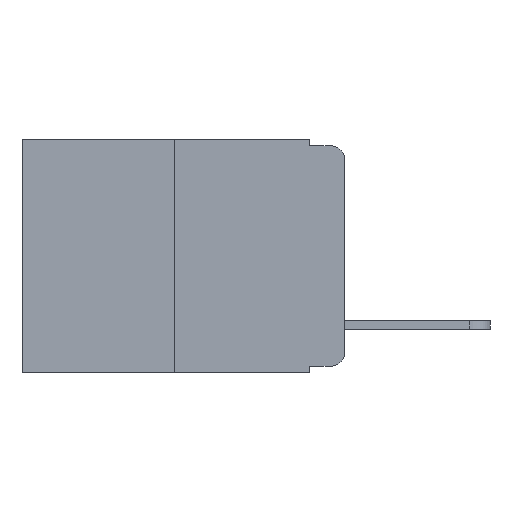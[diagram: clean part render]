
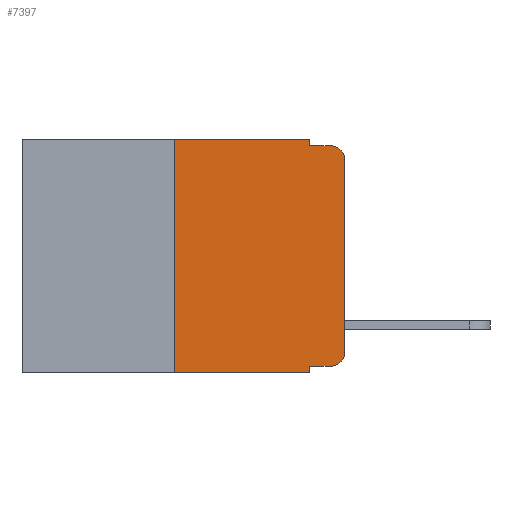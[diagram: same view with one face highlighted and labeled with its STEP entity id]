
A CAD part, left-side view. The second image highlights one B-rep face of the part: STEP entity #7397.
In plain terms, the highlighted planar face has unit normal (-1, 0, 0).
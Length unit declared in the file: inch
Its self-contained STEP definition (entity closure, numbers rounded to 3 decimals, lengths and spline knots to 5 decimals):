
#75 = LINE ( 'NONE', #168, #11359 ) ;
#168 = CARTESIAN_POINT ( 'NONE',  ( 0., 0.051, -0.333 ) ) ;
#244 = LINE ( 'NONE', #7957, #292 ) ;
#292 = VECTOR ( 'NONE', #8875, 39.37008 ) ;
#838 = VERTEX_POINT ( 'NONE', #10500 ) ;
#1460 = CARTESIAN_POINT ( 'NONE',  ( 0., 0., -0.313 ) ) ;
#1506 = EDGE_CURVE ( 'NONE', #4742, #7290, #4021, .T. ) ;
#1530 = ORIENTED_EDGE ( 'NONE', *, *, #1506, .T. ) ;
#1677 = ORIENTED_EDGE ( 'NONE', *, *, #1721, .T. ) ;
#1721 = EDGE_CURVE ( 'NONE', #7290, #1824, #3068, .T. ) ;
#1792 = ORIENTED_EDGE ( 'NONE', *, *, #2187, .F. ) ;
#1824 = VERTEX_POINT ( 'NONE', #8530 ) ;
#1874 = ORIENTED_EDGE ( 'NONE', *, *, #3678, .F. ) ;
#1945 = VERTEX_POINT ( 'NONE', #7128 ) ;
#1967 = ORIENTED_EDGE ( 'NONE', *, *, #5667, .F. ) ;
#2128 = ORIENTED_EDGE ( 'NONE', *, *, #4092, .F. ) ;
#2187 = EDGE_CURVE ( 'NONE', #7816, #1824, #11665, .T. ) ;
#2367 = ORIENTED_EDGE ( 'NONE', *, *, #3407, .T. ) ;
#2458 = ORIENTED_EDGE ( 'NONE', *, *, #4183, .F. ) ;
#2463 = CARTESIAN_POINT ( 'NONE',  ( 0., 0.051, 0. ) ) ;
#2758 = ORIENTED_EDGE ( 'NONE', *, *, #4461, .T. ) ;
#2759 = DIRECTION ( 'NONE',  ( -1., 0., 0. ) ) ;
#2853 = ORIENTED_EDGE ( 'NONE', *, *, #4691, .T. ) ;
#2864 = VECTOR ( 'NONE', #7560, 39.37008 ) ;
#3068 = CIRCLE ( 'NONE', #10586, 0.02 ) ;
#3407 = EDGE_CURVE ( 'NONE', #5128, #838, #244, .T. ) ;
#3635 = VECTOR ( 'NONE', #12746, 39.37008 ) ;
#3678 = EDGE_CURVE ( 'NONE', #10575, #7816, #6460, .T. ) ;
#3690 = VERTEX_POINT ( 'NONE', #12402 ) ;
#3712 = DIRECTION ( 'NONE',  ( 0., 0., 1. ) ) ;
#3852 = CARTESIAN_POINT ( 'NONE',  ( 0., 0.051, -0.01 ) ) ;
#4005 = VECTOR ( 'NONE', #10206, 39.37008 ) ;
#4021 = LINE ( 'NONE', #9619, #4005 ) ;
#4092 = EDGE_CURVE ( 'NONE', #5128, #6101, #4335, .T. ) ;
#4183 = EDGE_CURVE ( 'NONE', #1945, #838, #8688, .T. ) ;
#4283 = VECTOR ( 'NONE', #9826, 39.37008 ) ;
#4335 = LINE ( 'NONE', #7311, #4657 ) ;
#4381 = DIRECTION ( 'NONE',  ( 0., 0., -1. ) ) ;
#4461 = EDGE_CURVE ( 'NONE', #1945, #3690, #75, .T. ) ;
#4657 = VECTOR ( 'NONE', #3712, 39.37008 ) ;
#4691 = EDGE_CURVE ( 'NONE', #3690, #4742, #9610, .T. ) ;
#4742 = VERTEX_POINT ( 'NONE', #1460 ) ;
#4970 = CARTESIAN_POINT ( 'NONE',  ( 0., 0.25, -0.343 ) ) ;
#5128 = VERTEX_POINT ( 'NONE', #4970 ) ;
#5667 = EDGE_CURVE ( 'NONE', #6101, #10575, #9877, .T. ) ;
#6101 = VERTEX_POINT ( 'NONE', #12048 ) ;
#6220 = EDGE_LOOP ( 'NONE', ( #1530, #1677, #1792, #1874, #1967, #2128, #2367, #2458, #2758, #2853 ) ) ;
#6311 = AXIS2_PLACEMENT_3D ( 'NONE', #10920, #2759, #4381 ) ;
#6451 = DIRECTION ( 'NONE',  ( 0., -1., 0. ) ) ;
#6460 = LINE ( 'NONE', #2463, #3635 ) ;
#7128 = CARTESIAN_POINT ( 'NONE',  ( 0., 0.051, -0.333 ) ) ;
#7256 = DIRECTION ( 'NONE',  ( 0., -1., 0. ) ) ;
#7290 = VERTEX_POINT ( 'NONE', #12981 ) ;
#7311 = CARTESIAN_POINT ( 'NONE',  ( 0., 0.25, 0. ) ) ;
#7397 = ADVANCED_FACE ( 'NONE', ( #7904 ), #11223, .F. ) ;
#7560 = DIRECTION ( 'NONE',  ( 0., 0., -1. ) ) ;
#7816 = VERTEX_POINT ( 'NONE', #3852 ) ;
#7904 = FACE_OUTER_BOUND ( 'NONE', #6220, .T. ) ;
#7957 = CARTESIAN_POINT ( 'NONE',  ( 0., 0.473, -0.343 ) ) ;
#8482 = DIRECTION ( 'NONE',  ( 0., 0., -1. ) ) ;
#8486 = DIRECTION ( 'NONE',  ( -1., 0., 0. ) ) ;
#8530 = CARTESIAN_POINT ( 'NONE',  ( 0., 0.02, -0.01 ) ) ;
#8688 = LINE ( 'NONE', #9442, #2864 ) ;
#8875 = DIRECTION ( 'NONE',  ( 0., -1., 0. ) ) ;
#9058 = CARTESIAN_POINT ( 'NONE',  ( 0., 0.02, -0.03 ) ) ;
#9442 = CARTESIAN_POINT ( 'NONE',  ( 0., 0.051, 0. ) ) ;
#9610 = CIRCLE ( 'NONE', #6311, 0.02 ) ;
#9619 = CARTESIAN_POINT ( 'NONE',  ( 0., 0., 0. ) ) ;
#9624 = CARTESIAN_POINT ( 'NONE',  ( 0., 0.473, 0. ) ) ;
#9729 = CARTESIAN_POINT ( 'NONE',  ( 0., 0.051, 0. ) ) ;
#9793 = CARTESIAN_POINT ( 'NONE',  ( 0., 0.051, -0.01 ) ) ;
#9826 = DIRECTION ( 'NONE',  ( 0., -1., 0. ) ) ;
#9877 = LINE ( 'NONE', #9624, #4283 ) ;
#10206 = DIRECTION ( 'NONE',  ( 0., 0., 1. ) ) ;
#10301 = AXIS2_PLACEMENT_3D ( 'NONE', #11524, #11192, #11181 ) ;
#10500 = CARTESIAN_POINT ( 'NONE',  ( 0., 0.051, -0.343 ) ) ;
#10575 = VERTEX_POINT ( 'NONE', #9729 ) ;
#10586 = AXIS2_PLACEMENT_3D ( 'NONE', #9058, #8486, #8482 ) ;
#10920 = CARTESIAN_POINT ( 'NONE',  ( 0., 0.02, -0.313 ) ) ;
#11181 = DIRECTION ( 'NONE',  ( 0., 0., -1. ) ) ;
#11192 = DIRECTION ( 'NONE',  ( 1., 0., 0. ) ) ;
#11223 = PLANE ( 'NONE',  #10301 ) ;
#11359 = VECTOR ( 'NONE', #6451, 39.37008 ) ;
#11502 = VECTOR ( 'NONE', #7256, 39.37008 ) ;
#11524 = CARTESIAN_POINT ( 'NONE',  ( 0., 0.473, 0. ) ) ;
#11665 = LINE ( 'NONE', #9793, #11502 ) ;
#12048 = CARTESIAN_POINT ( 'NONE',  ( 0., 0.25, 0. ) ) ;
#12402 = CARTESIAN_POINT ( 'NONE',  ( 0., 0.02, -0.333 ) ) ;
#12746 = DIRECTION ( 'NONE',  ( 0., 0., -1. ) ) ;
#12981 = CARTESIAN_POINT ( 'NONE',  ( 0., 0., -0.03 ) ) ;
